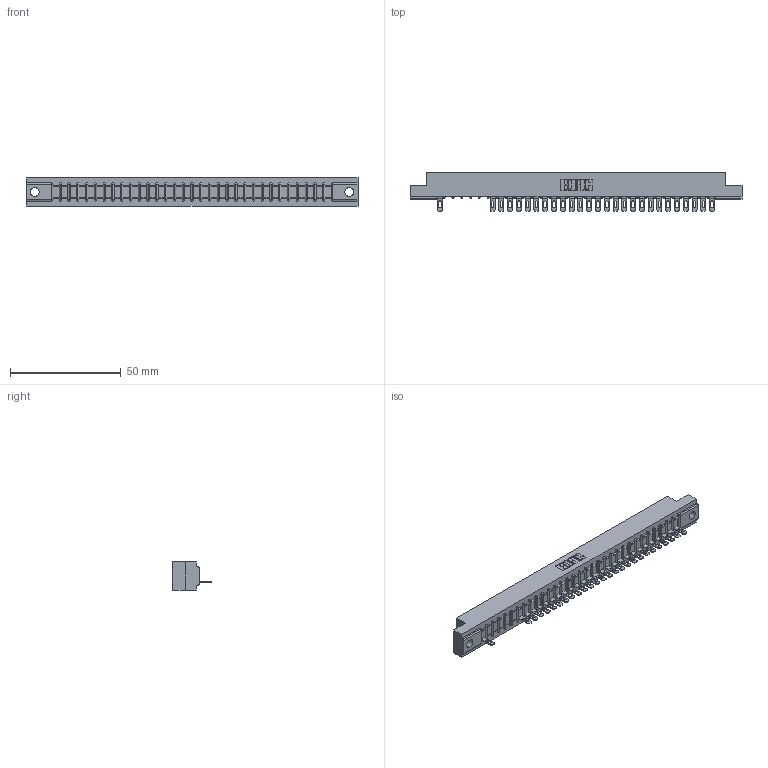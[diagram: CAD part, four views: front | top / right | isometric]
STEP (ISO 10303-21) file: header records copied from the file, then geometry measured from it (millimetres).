
FILE_DESCRIPTION (( 'STEP AP203' ), '1' );
FILE_NAME ('357-032-501-104.STEP', '2018-08-09T23:35:21', ( '' ), ( '' ), 'SwSTEP 2.0', 'SolidWorks 2016', '' );
FILE_SCHEMA (( 'CONFIG_CONTROL_DESIGN' ));
Length unit declared in the file: inch
Products named in the file (3): 307 Part_.156 Dia Mounting Holes; 307-290-002_501; 357-032-501-104
Assembly tree (28 placements, depth 2):
  357-032-501-104
    307 Part_.156 Dia Mounting Holes
    307-290-002_501  x27
Bounding box: 149.81 x 17.42 x 12.7 mm (x, y, z)
Volume: 15729.8 mm3; surface area: 18650.5 mm2
Topology: 28 solids, 28 shells, 2317 faces, 7105 edges, 4646 vertices
Faces by surface type: plane 1332, cylinder 919, sphere 66
Entity records: 29718 total; most frequent: CARTESIAN_POINT 5037, ORIENTED_EDGE 5030, DIRECTION 4889, EDGE_CURVE 2515, VECTOR 1925, LINE 1925, VERTEX_POINT 1630, AXIS2_PLACEMENT_3D 1482
